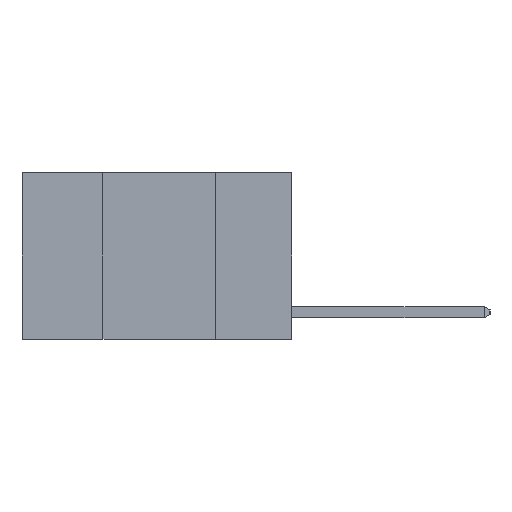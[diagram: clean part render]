
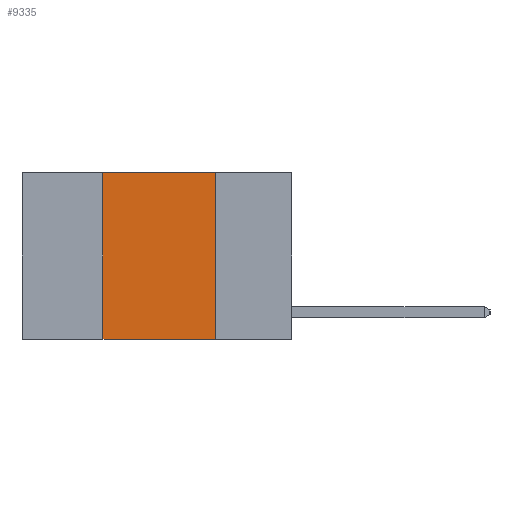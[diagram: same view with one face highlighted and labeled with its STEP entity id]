
A CAD part, left-side view. The second image highlights one B-rep face of the part: STEP entity #9335.
In plain terms, the highlighted planar face has unit normal (-1, 0, 0).
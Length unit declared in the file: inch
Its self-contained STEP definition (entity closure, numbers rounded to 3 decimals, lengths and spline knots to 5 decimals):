
#474 = DIRECTION ( 'NONE',  ( 0., 0., 1. ) ) ;
#706 = FACE_OUTER_BOUND ( 'NONE', #6747, .T. ) ;
#827 = DIRECTION ( 'NONE',  ( 0., -1., 0. ) ) ;
#854 = CARTESIAN_POINT ( 'NONE',  ( 0., 0.6, 0. ) ) ;
#1250 = VECTOR ( 'NONE', #2924, 39.37008 ) ;
#1366 = VECTOR ( 'NONE', #474, 39.37008 ) ;
#1594 = DIRECTION ( 'NONE',  ( 0., 0., -1. ) ) ;
#1689 = VERTEX_POINT ( 'NONE', #2696 ) ;
#1950 = ORIENTED_EDGE ( 'NONE', *, *, #9294, .F. ) ;
#2166 = EDGE_CURVE ( 'NONE', #3903, #5229, #7453, .T. ) ;
#2404 = EDGE_CURVE ( 'NONE', #3903, #3619, #4931, .T. ) ;
#2600 = CARTESIAN_POINT ( 'NONE',  ( 0., 0.42, 0. ) ) ;
#2626 = LINE ( 'NONE', #5242, #4832 ) ;
#2629 = DIRECTION ( 'NONE',  ( 0., 0., -1. ) ) ;
#2696 = CARTESIAN_POINT ( 'NONE',  ( 0., 0.17, 0. ) ) ;
#2799 = CARTESIAN_POINT ( 'NONE',  ( 0., 0.17, -0.37 ) ) ;
#2924 = DIRECTION ( 'NONE',  ( 0., -1., 0. ) ) ;
#3443 = ORIENTED_EDGE ( 'NONE', *, *, #2166, .F. ) ;
#3619 = VERTEX_POINT ( 'NONE', #2799 ) ;
#3903 = VERTEX_POINT ( 'NONE', #4714 ) ;
#4029 = EDGE_CURVE ( 'NONE', #1689, #3619, #7436, .T. ) ;
#4714 = CARTESIAN_POINT ( 'NONE',  ( 0., 0.42, -0.37 ) ) ;
#4832 = VECTOR ( 'NONE', #827, 39.37008 ) ;
#4931 = LINE ( 'NONE', #6603, #1250 ) ;
#5229 = VERTEX_POINT ( 'NONE', #8611 ) ;
#5242 = CARTESIAN_POINT ( 'NONE',  ( 0., 0.6, 0. ) ) ;
#5274 = PLANE ( 'NONE',  #9080 ) ;
#5884 = ORIENTED_EDGE ( 'NONE', *, *, #2404, .T. ) ;
#5995 = DIRECTION ( 'NONE',  ( 1., 0., 0. ) ) ;
#6324 = CARTESIAN_POINT ( 'NONE',  ( 0., 0.17, 0. ) ) ;
#6603 = CARTESIAN_POINT ( 'NONE',  ( 0., 0.6, -0.37 ) ) ;
#6747 = EDGE_LOOP ( 'NONE', ( #8847, #1950, #3443, #5884 ) ) ;
#7203 = VECTOR ( 'NONE', #2629, 39.37008 ) ;
#7436 = LINE ( 'NONE', #6324, #7203 ) ;
#7453 = LINE ( 'NONE', #2600, #1366 ) ;
#8611 = CARTESIAN_POINT ( 'NONE',  ( 0., 0.42, 0. ) ) ;
#8847 = ORIENTED_EDGE ( 'NONE', *, *, #4029, .F. ) ;
#9080 = AXIS2_PLACEMENT_3D ( 'NONE', #854, #5995, #1594 ) ;
#9294 = EDGE_CURVE ( 'NONE', #5229, #1689, #2626, .T. ) ;
#9335 = ADVANCED_FACE ( 'NONE', ( #706 ), #5274, .F. ) ;
